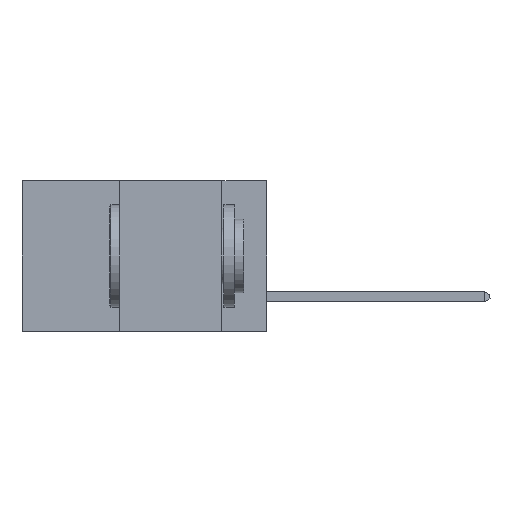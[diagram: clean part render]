
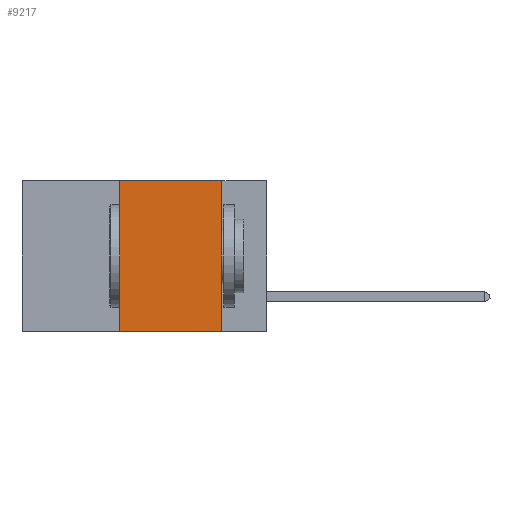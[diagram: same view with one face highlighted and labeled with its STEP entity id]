
A CAD part, left-side view. The second image highlights one B-rep face of the part: STEP entity #9217.
In plain terms, the highlighted planar face has unit normal (-1, 0, 0).
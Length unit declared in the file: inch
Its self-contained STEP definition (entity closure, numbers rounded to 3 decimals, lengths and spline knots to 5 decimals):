
#63 = EDGE_CURVE ( 'NONE', #6918, #4332, #4538, .T. ) ;
#581 = DIRECTION ( 'NONE',  ( 0., -1., 0. ) ) ;
#659 = VECTOR ( 'NONE', #581, 39.37008 ) ;
#678 = EDGE_CURVE ( 'NONE', #6034, #9152, #8340, .T. ) ;
#947 = VECTOR ( 'NONE', #6190, 39.37008 ) ;
#1403 = CARTESIAN_POINT ( 'NONE',  ( 0., 0.36, 0. ) ) ;
#1479 = EDGE_CURVE ( 'NONE', #4332, #6034, #2571, .T. ) ;
#1771 = CARTESIAN_POINT ( 'NONE',  ( 0., 0.36, 0. ) ) ;
#1779 = CARTESIAN_POINT ( 'NONE',  ( 0., 0.6, 0. ) ) ;
#2242 = ORIENTED_EDGE ( 'NONE', *, *, #4400, .T. ) ;
#2571 = LINE ( 'NONE', #1779, #947 ) ;
#2581 = VECTOR ( 'NONE', #4405, 39.37008 ) ;
#2704 = VECTOR ( 'NONE', #3806, 39.37008 ) ;
#2968 = CARTESIAN_POINT ( 'NONE',  ( 0., 0.11, -0.37 ) ) ;
#3580 = DIRECTION ( 'NONE',  ( 0., 0., -1. ) ) ;
#3689 = EDGE_LOOP ( 'NONE', ( #5806, #7421, #7824, #2242 ) ) ;
#3806 = DIRECTION ( 'NONE',  ( 0., 0., -1. ) ) ;
#4332 = VERTEX_POINT ( 'NONE', #1771 ) ;
#4353 = DIRECTION ( 'NONE',  ( 1., 0., 0. ) ) ;
#4400 = EDGE_CURVE ( 'NONE', #6918, #9152, #5165, .T. ) ;
#4405 = DIRECTION ( 'NONE',  ( 0., 0., 1. ) ) ;
#4538 = LINE ( 'NONE', #1403, #2581 ) ;
#4605 = CARTESIAN_POINT ( 'NONE',  ( 0., 0.11, 0. ) ) ;
#5165 = LINE ( 'NONE', #5636, #659 ) ;
#5636 = CARTESIAN_POINT ( 'NONE',  ( 0., 0.6, -0.37 ) ) ;
#5760 = CARTESIAN_POINT ( 'NONE',  ( 0., 0.6, 0. ) ) ;
#5806 = ORIENTED_EDGE ( 'NONE', *, *, #678, .F. ) ;
#5989 = CARTESIAN_POINT ( 'NONE',  ( 0., 0.11, 0. ) ) ;
#6034 = VERTEX_POINT ( 'NONE', #4605 ) ;
#6190 = DIRECTION ( 'NONE',  ( 0., -1., 0. ) ) ;
#6599 = PLANE ( 'NONE',  #9041 ) ;
#6918 = VERTEX_POINT ( 'NONE', #7878 ) ;
#7421 = ORIENTED_EDGE ( 'NONE', *, *, #1479, .F. ) ;
#7824 = ORIENTED_EDGE ( 'NONE', *, *, #63, .F. ) ;
#7878 = CARTESIAN_POINT ( 'NONE',  ( 0., 0.36, -0.37 ) ) ;
#8340 = LINE ( 'NONE', #5989, #2704 ) ;
#8570 = FACE_OUTER_BOUND ( 'NONE', #3689, .T. ) ;
#9041 = AXIS2_PLACEMENT_3D ( 'NONE', #5760, #4353, #3580 ) ;
#9152 = VERTEX_POINT ( 'NONE', #2968 ) ;
#9217 = ADVANCED_FACE ( 'NONE', ( #8570 ), #6599, .F. ) ;
